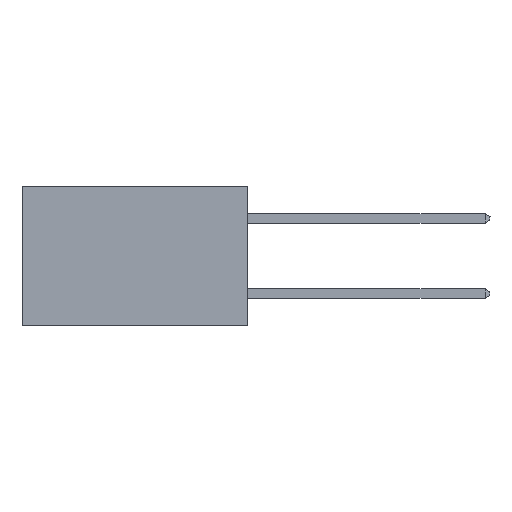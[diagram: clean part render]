
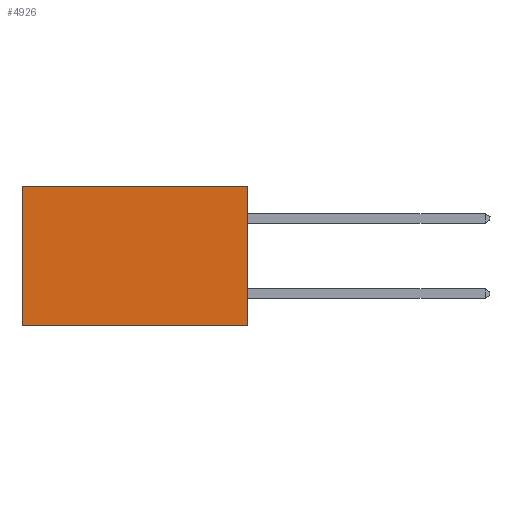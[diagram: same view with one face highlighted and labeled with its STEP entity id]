
A CAD part, left-side view. The second image highlights one B-rep face of the part: STEP entity #4926.
In plain terms, the highlighted planar face has unit normal (-1, 0, 0).
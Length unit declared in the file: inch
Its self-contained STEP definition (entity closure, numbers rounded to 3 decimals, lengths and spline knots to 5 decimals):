
#151 = DIRECTION ( 'NONE',  ( 0., 1., 0. ) ) ;
#666 = ORIENTED_EDGE ( 'NONE', *, *, #18035, .T. ) ;
#744 = LINE ( 'NONE', #12046, #6023 ) ;
#1158 = VERTEX_POINT ( 'NONE', #23054 ) ;
#1211 = VERTEX_POINT ( 'NONE', #2004 ) ;
#1435 = EDGE_CURVE ( 'NONE', #13336, #12554, #744, .T. ) ;
#2004 = CARTESIAN_POINT ( 'NONE',  ( 0.298, 0.6, 0. ) ) ;
#2869 = CARTESIAN_POINT ( 'NONE',  ( 0.298, 0.6, 0. ) ) ;
#3032 = CARTESIAN_POINT ( 'NONE',  ( 0.298, 0., -0.37 ) ) ;
#4926 = ADVANCED_FACE ( 'NONE', ( #6280 ), #13455, .F. ) ;
#6023 = VECTOR ( 'NONE', #12300, 39.37008 ) ;
#6280 = FACE_OUTER_BOUND ( 'NONE', #8659, .T. ) ;
#7645 = ORIENTED_EDGE ( 'NONE', *, *, #1435, .F. ) ;
#8659 = EDGE_LOOP ( 'NONE', ( #666, #19922, #7645, #12287 ) ) ;
#12046 = CARTESIAN_POINT ( 'NONE',  ( 0.298, 0., 0. ) ) ;
#12287 = ORIENTED_EDGE ( 'NONE', *, *, #14565, .T. ) ;
#12300 = DIRECTION ( 'NONE',  ( 0., 0., -1. ) ) ;
#12554 = VERTEX_POINT ( 'NONE', #13560 ) ;
#12657 = VECTOR ( 'NONE', #151, 39.37008 ) ;
#12808 = DIRECTION ( 'NONE',  ( 0., 1., 0. ) ) ;
#13336 = VERTEX_POINT ( 'NONE', #14301 ) ;
#13455 = PLANE ( 'NONE',  #18595 ) ;
#13560 = CARTESIAN_POINT ( 'NONE',  ( 0.298, 0., -0.37 ) ) ;
#14301 = CARTESIAN_POINT ( 'NONE',  ( 0.298, 0., 0. ) ) ;
#14565 = EDGE_CURVE ( 'NONE', #13336, #1211, #22917, .T. ) ;
#15050 = VECTOR ( 'NONE', #18514, 39.37008 ) ;
#16509 = CARTESIAN_POINT ( 'NONE',  ( 0.298, 0., 0. ) ) ;
#17225 = DIRECTION ( 'NONE',  ( 0., 0., -1. ) ) ;
#18035 = EDGE_CURVE ( 'NONE', #1211, #1158, #19556, .T. ) ;
#18092 = EDGE_CURVE ( 'NONE', #12554, #1158, #23443, .T. ) ;
#18514 = DIRECTION ( 'NONE',  ( 0., 0., -1. ) ) ;
#18595 = AXIS2_PLACEMENT_3D ( 'NONE', #16509, #22954, #17225 ) ;
#19556 = LINE ( 'NONE', #2869, #15050 ) ;
#19922 = ORIENTED_EDGE ( 'NONE', *, *, #18092, .F. ) ;
#22836 = VECTOR ( 'NONE', #12808, 39.37008 ) ;
#22917 = LINE ( 'NONE', #23489, #12657 ) ;
#22954 = DIRECTION ( 'NONE',  ( 1., 0., 0. ) ) ;
#23054 = CARTESIAN_POINT ( 'NONE',  ( 0.298, 0.6, -0.37 ) ) ;
#23443 = LINE ( 'NONE', #3032, #22836 ) ;
#23489 = CARTESIAN_POINT ( 'NONE',  ( 0.298, 0., 0. ) ) ;
